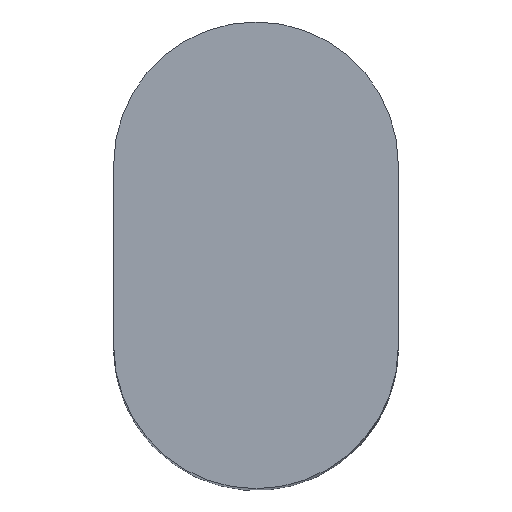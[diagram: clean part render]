
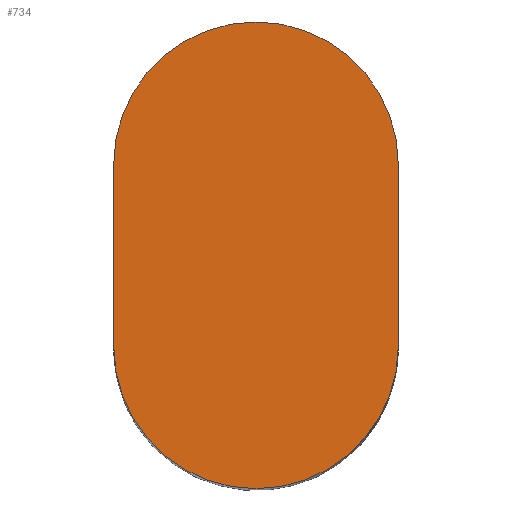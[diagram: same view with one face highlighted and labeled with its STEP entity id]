
A CAD part, top view. The second image highlights one B-rep face of the part: STEP entity #734.
In plain terms, the highlighted planar face has unit normal (0, 0, 1).
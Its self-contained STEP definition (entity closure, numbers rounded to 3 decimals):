
#5 = EDGE_LOOP ( 'NONE', ( #1131, #724, #1048, #874 ) ) ;
#18 = CARTESIAN_POINT ( 'NONE',  ( -15., 27.969, 60. ) ) ;
#24 = AXIS2_PLACEMENT_3D ( 'NONE', #1034, #859, #230 ) ;
#96 = CARTESIAN_POINT ( 'NONE',  ( 0., 27.969, 60. ) ) ;
#119 = LINE ( 'NONE', #642, #1049 ) ;
#132 = DIRECTION ( 'NONE',  ( 0., 0., 1. ) ) ;
#170 = VERTEX_POINT ( 'NONE', #1001 ) ;
#179 = VERTEX_POINT ( 'NONE', #18 ) ;
#230 = DIRECTION ( 'NONE',  ( 1., 0., 0. ) ) ;
#321 = LINE ( 'NONE', #412, #358 ) ;
#358 = VECTOR ( 'NONE', #928, 1000. ) ;
#364 = DIRECTION ( 'NONE',  ( 0., 1., 0. ) ) ;
#412 = CARTESIAN_POINT ( 'NONE',  ( -15., 47.167, 60. ) ) ;
#576 = FACE_OUTER_BOUND ( 'NONE', #5, .T. ) ;
#582 = PLANE ( 'NONE',  #996 ) ;
#619 = CIRCLE ( 'NONE', #1126, 15. ) ;
#642 = CARTESIAN_POINT ( 'NONE',  ( 15., 27.969, 60. ) ) ;
#657 = VERTEX_POINT ( 'NONE', #1121 ) ;
#659 = CARTESIAN_POINT ( 'NONE',  ( 15., 47.167, 60. ) ) ;
#661 = EDGE_CURVE ( 'NONE', #170, #179, #321, .T. ) ;
#715 = VERTEX_POINT ( 'NONE', #659 ) ;
#724 = ORIENTED_EDGE ( 'NONE', *, *, #661, .T. ) ;
#734 = ADVANCED_FACE ( 'NONE', ( #576 ), #582, .T. ) ;
#744 = EDGE_CURVE ( 'NONE', #715, #170, #1091, .T. ) ;
#844 = DIRECTION ( 'NONE',  ( 1., 0., 0. ) ) ;
#859 = DIRECTION ( 'NONE',  ( 0., 0., 1. ) ) ;
#874 = ORIENTED_EDGE ( 'NONE', *, *, #909, .T. ) ;
#909 = EDGE_CURVE ( 'NONE', #657, #715, #119, .T. ) ;
#924 = CARTESIAN_POINT ( 'NONE',  ( 0., 47.167, 60. ) ) ;
#928 = DIRECTION ( 'NONE',  ( 0., -1., 0. ) ) ;
#948 = EDGE_CURVE ( 'NONE', #179, #657, #619, .T. ) ;
#986 = DIRECTION ( 'NONE',  ( 0., 0., 1. ) ) ;
#996 = AXIS2_PLACEMENT_3D ( 'NONE', #924, #132, #844 ) ;
#1001 = CARTESIAN_POINT ( 'NONE',  ( -15., 47.167, 60. ) ) ;
#1034 = CARTESIAN_POINT ( 'NONE',  ( 0., 47.167, 60. ) ) ;
#1048 = ORIENTED_EDGE ( 'NONE', *, *, #948, .T. ) ;
#1049 = VECTOR ( 'NONE', #364, 1000. ) ;
#1084 = DIRECTION ( 'NONE',  ( 1., 0., 0. ) ) ;
#1091 = CIRCLE ( 'NONE', #24, 15. ) ;
#1121 = CARTESIAN_POINT ( 'NONE',  ( 15., 27.969, 60. ) ) ;
#1126 = AXIS2_PLACEMENT_3D ( 'NONE', #96, #986, #1084 ) ;
#1131 = ORIENTED_EDGE ( 'NONE', *, *, #744, .T. ) ;
